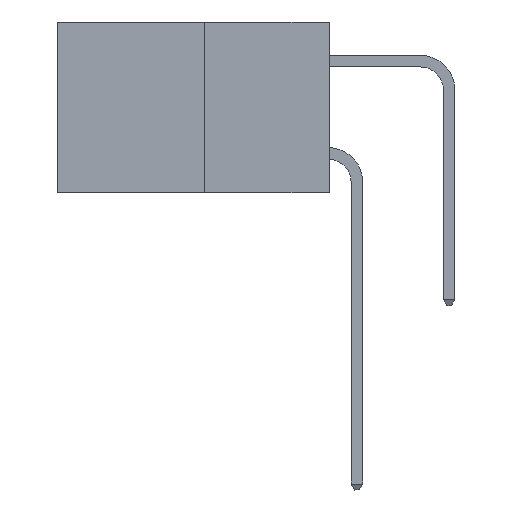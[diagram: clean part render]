
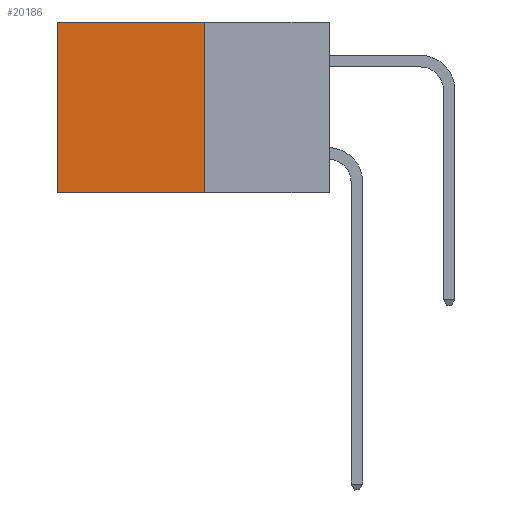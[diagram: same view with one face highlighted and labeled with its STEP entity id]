
A CAD part, left-side view. The second image highlights one B-rep face of the part: STEP entity #20186.
In plain terms, the highlighted planar face has unit normal (-1, 0, 0).
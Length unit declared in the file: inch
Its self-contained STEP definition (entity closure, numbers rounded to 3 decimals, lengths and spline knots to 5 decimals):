
#899 = DIRECTION ( 'NONE',  ( 0., 0., -1. ) ) ;
#982 = CARTESIAN_POINT ( 'NONE',  ( 0.277, 0.59, -0.37 ) ) ;
#1290 = DIRECTION ( 'NONE',  ( 0., 0., -1. ) ) ;
#1427 = CARTESIAN_POINT ( 'NONE',  ( 0.277, 0.27, 0. ) ) ;
#1669 = LINE ( 'NONE', #982, #8084 ) ;
#2137 = LINE ( 'NONE', #7021, #17065 ) ;
#4263 = VECTOR ( 'NONE', #21739, 39.37008 ) ;
#5952 = EDGE_LOOP ( 'NONE', ( #21429, #17319, #18888, #20958 ) ) ;
#6785 = CARTESIAN_POINT ( 'NONE',  ( 0.277, 0.27, -0.37 ) ) ;
#7021 = CARTESIAN_POINT ( 'NONE',  ( 0.277, 0.27, -0.37 ) ) ;
#7106 = PLANE ( 'NONE',  #13059 ) ;
#7909 = CARTESIAN_POINT ( 'NONE',  ( 0.277, 0.59, 0. ) ) ;
#8084 = VECTOR ( 'NONE', #899, 39.37008 ) ;
#8200 = CARTESIAN_POINT ( 'NONE',  ( 0.277, 0.27, -0.37 ) ) ;
#8394 = VECTOR ( 'NONE', #12653, 39.37008 ) ;
#9323 = EDGE_CURVE ( 'NONE', #12386, #18536, #19153, .T. ) ;
#12141 = EDGE_CURVE ( 'NONE', #24804, #18536, #1669, .T. ) ;
#12386 = VERTEX_POINT ( 'NONE', #6785 ) ;
#12653 = DIRECTION ( 'NONE',  ( 0., 1., 0. ) ) ;
#12903 = EDGE_CURVE ( 'NONE', #20929, #24804, #13573, .T. ) ;
#12976 = DIRECTION ( 'NONE',  ( 1., 0., 0. ) ) ;
#13059 = AXIS2_PLACEMENT_3D ( 'NONE', #18750, #12976, #1290 ) ;
#13573 = LINE ( 'NONE', #20323, #8394 ) ;
#17065 = VECTOR ( 'NONE', #22487, 39.37008 ) ;
#17319 = ORIENTED_EDGE ( 'NONE', *, *, #9323, .F. ) ;
#18536 = VERTEX_POINT ( 'NONE', #25094 ) ;
#18750 = CARTESIAN_POINT ( 'NONE',  ( 0.277, 0.27, -0.37 ) ) ;
#18888 = ORIENTED_EDGE ( 'NONE', *, *, #20149, .F. ) ;
#19153 = LINE ( 'NONE', #8200, #4263 ) ;
#20149 = EDGE_CURVE ( 'NONE', #20929, #12386, #2137, .T. ) ;
#20186 = ADVANCED_FACE ( 'NONE', ( #21560 ), #7106, .F. ) ;
#20323 = CARTESIAN_POINT ( 'NONE',  ( 0.277, 0.27, 0. ) ) ;
#20929 = VERTEX_POINT ( 'NONE', #1427 ) ;
#20958 = ORIENTED_EDGE ( 'NONE', *, *, #12903, .T. ) ;
#21429 = ORIENTED_EDGE ( 'NONE', *, *, #12141, .T. ) ;
#21560 = FACE_OUTER_BOUND ( 'NONE', #5952, .T. ) ;
#21739 = DIRECTION ( 'NONE',  ( 0., 1., 0. ) ) ;
#22487 = DIRECTION ( 'NONE',  ( 0., 0., -1. ) ) ;
#24804 = VERTEX_POINT ( 'NONE', #7909 ) ;
#25094 = CARTESIAN_POINT ( 'NONE',  ( 0.277, 0.59, -0.37 ) ) ;
